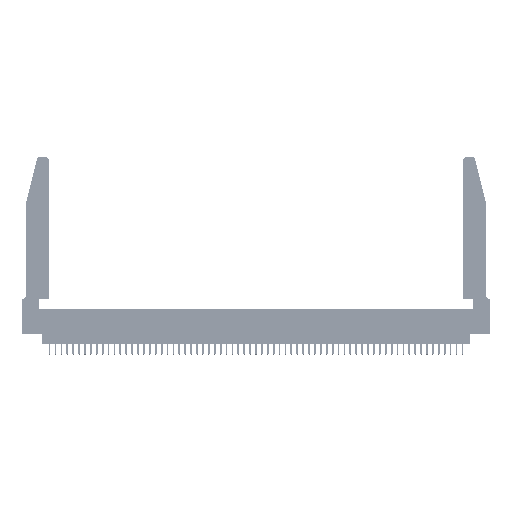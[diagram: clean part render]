
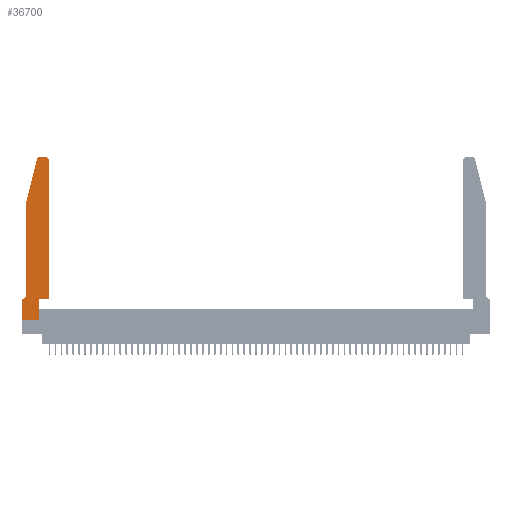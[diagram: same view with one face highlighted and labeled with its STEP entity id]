
A CAD part, top view. The second image highlights one B-rep face of the part: STEP entity #36700.
In plain terms, the highlighted planar face has unit normal (0, 0, 1).
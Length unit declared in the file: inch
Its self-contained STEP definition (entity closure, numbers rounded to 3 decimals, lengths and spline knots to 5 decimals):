
#953 = CARTESIAN_POINT ( 'NONE',  ( 0.2865, 0.35, 0.37 ) ) ;
#1869 = DIRECTION ( 'NONE',  ( 0., 0., 1. ) ) ;
#2263 = ORIENTED_EDGE ( 'NONE', *, *, #51978, .T. ) ;
#2476 = CARTESIAN_POINT ( 'NONE',  ( 0.0755, 2., 0.37 ) ) ;
#2962 = EDGE_CURVE ( 'NONE', #43943, #24867, #7674, .T. ) ;
#3345 = LINE ( 'NONE', #11328, #40398 ) ;
#3544 = EDGE_CURVE ( 'NONE', #31017, #8920, #23420, .T. ) ;
#3588 = VERTEX_POINT ( 'NONE', #51928 ) ;
#3883 = LINE ( 'NONE', #42548, #52692 ) ;
#4078 = ORIENTED_EDGE ( 'NONE', *, *, #52230, .T. ) ;
#4476 = LINE ( 'NONE', #19630, #51867 ) ;
#6431 = EDGE_LOOP ( 'NONE', ( #4078, #2263, #52543, #18265, #25940, #31523, #36903, #30570, #8687, #23156, #23454, #7984 ) ) ;
#7514 = AXIS2_PLACEMENT_3D ( 'NONE', #26543, #22287, #53197 ) ;
#7674 = LINE ( 'NONE', #29128, #52996 ) ;
#7984 = ORIENTED_EDGE ( 'NONE', *, *, #49078, .T. ) ;
#8687 = ORIENTED_EDGE ( 'NONE', *, *, #38161, .T. ) ;
#8920 = VERTEX_POINT ( 'NONE', #56820 ) ;
#10149 = AXIS2_PLACEMENT_3D ( 'NONE', #55018, #1869, #24113 ) ;
#10168 = AXIS2_PLACEMENT_3D ( 'NONE', #50578, #32696, #54780 ) ;
#10379 = VECTOR ( 'NONE', #34046, 39.37008 ) ;
#10678 = DIRECTION ( 'NONE',  ( 1., 0., 0. ) ) ;
#11328 = CARTESIAN_POINT ( 'NONE',  ( 0.2865, 0.35, 0.37 ) ) ;
#12524 = EDGE_CURVE ( 'NONE', #33496, #15859, #43593, .T. ) ;
#12536 = EDGE_CURVE ( 'NONE', #15859, #3588, #37429, .T. ) ;
#14085 = CARTESIAN_POINT ( 'NONE',  ( 0., 0., 0.37 ) ) ;
#14620 = AXIS2_PLACEMENT_3D ( 'NONE', #32933, #36957, #10678 ) ;
#14712 = VERTEX_POINT ( 'NONE', #953 ) ;
#15438 = EDGE_CURVE ( 'NONE', #22731, #39169, #36406, .T. ) ;
#15859 = VERTEX_POINT ( 'NONE', #52670 ) ;
#15919 = CARTESIAN_POINT ( 'NONE',  ( 0.2865, 0., 0.37 ) ) ;
#17232 = FACE_OUTER_BOUND ( 'NONE', #6431, .T. ) ;
#17410 = EDGE_CURVE ( 'NONE', #14712, #31017, #3883, .T. ) ;
#17604 = CARTESIAN_POINT ( 'NONE',  ( 0.0755, 0.42, 0.37 ) ) ;
#18265 = ORIENTED_EDGE ( 'NONE', *, *, #39097, .T. ) ;
#18310 = CIRCLE ( 'NONE', #10168, 0.03 ) ;
#19630 = CARTESIAN_POINT ( 'NONE',  ( 0., 0., 0.37 ) ) ;
#22086 = VERTEX_POINT ( 'NONE', #50207 ) ;
#22287 = DIRECTION ( 'NONE',  ( 0., 0., -1. ) ) ;
#22731 = VERTEX_POINT ( 'NONE', #14085 ) ;
#23156 = ORIENTED_EDGE ( 'NONE', *, *, #17410, .T. ) ;
#23420 = LINE ( 'NONE', #29648, #10379 ) ;
#23454 = ORIENTED_EDGE ( 'NONE', *, *, #3544, .T. ) ;
#24026 = DIRECTION ( 'NONE',  ( 0., -1., 0. ) ) ;
#24113 = DIRECTION ( 'NONE',  ( 1., 0., 0. ) ) ;
#24546 = DIRECTION ( 'NONE',  ( 0., -1., 0. ) ) ;
#24754 = VECTOR ( 'NONE', #36559, 39.37008 ) ;
#24758 = DIRECTION ( 'NONE',  ( 0., 1., 0. ) ) ;
#24867 = VERTEX_POINT ( 'NONE', #30318 ) ;
#25940 = ORIENTED_EDGE ( 'NONE', *, *, #12524, .T. ) ;
#26391 = CARTESIAN_POINT ( 'NONE',  ( 0.2605, 2.75, 0.37 ) ) ;
#26543 = CARTESIAN_POINT ( 'NONE',  ( 0.0055, 0.42, 0.37 ) ) ;
#26551 = VECTOR ( 'NONE', #24546, 39.37008 ) ;
#27164 = VECTOR ( 'NONE', #39371, 39.37008 ) ;
#28107 = CARTESIAN_POINT ( 'NONE',  ( 0.4505, 0.35, 0.37 ) ) ;
#28170 = PLANE ( 'NONE',  #10149 ) ;
#29128 = CARTESIAN_POINT ( 'NONE',  ( 0.0755, 2., 0.37 ) ) ;
#29648 = CARTESIAN_POINT ( 'NONE',  ( 0.4505, 0.35, 0.37 ) ) ;
#30318 = CARTESIAN_POINT ( 'NONE',  ( 0.0755, 2., 0.37 ) ) ;
#30570 = ORIENTED_EDGE ( 'NONE', *, *, #15438, .T. ) ;
#31017 = VERTEX_POINT ( 'NONE', #28107 ) ;
#31523 = ORIENTED_EDGE ( 'NONE', *, *, #12536, .T. ) ;
#32696 = DIRECTION ( 'NONE',  ( 0., 0., 1. ) ) ;
#32933 = CARTESIAN_POINT ( 'NONE',  ( 0.284, 2.72, 0.37 ) ) ;
#33095 = VERTEX_POINT ( 'NONE', #40467 ) ;
#33496 = VERTEX_POINT ( 'NONE', #17604 ) ;
#34046 = DIRECTION ( 'NONE',  ( 0., 1., 0. ) ) ;
#35190 = DIRECTION ( 'NONE',  ( -1., 0., 0. ) ) ;
#36406 = LINE ( 'NONE', #45381, #24754 ) ;
#36559 = DIRECTION ( 'NONE',  ( 1., 0., 0. ) ) ;
#36700 = ADVANCED_FACE ( 'NONE', ( #17232 ), #28170, .T. ) ;
#36903 = ORIENTED_EDGE ( 'NONE', *, *, #42087, .T. ) ;
#36957 = DIRECTION ( 'NONE',  ( 0., 0., 1. ) ) ;
#37429 = LINE ( 'NONE', #38436, #27164 ) ;
#38161 = EDGE_CURVE ( 'NONE', #39169, #14712, #3345, .T. ) ;
#38205 = LINE ( 'NONE', #2476, #26551 ) ;
#38436 = CARTESIAN_POINT ( 'NONE',  ( 0.0755, 0.35, 0.37 ) ) ;
#39097 = EDGE_CURVE ( 'NONE', #24867, #33496, #38205, .T. ) ;
#39169 = VERTEX_POINT ( 'NONE', #15919 ) ;
#39371 = DIRECTION ( 'NONE',  ( -1., 0., 0. ) ) ;
#40398 = VECTOR ( 'NONE', #24758, 39.37008 ) ;
#40467 = CARTESIAN_POINT ( 'NONE',  ( 0.284, 2.75, 0.37 ) ) ;
#42056 = VECTOR ( 'NONE', #35190, 39.37008 ) ;
#42087 = EDGE_CURVE ( 'NONE', #3588, #22731, #4476, .T. ) ;
#42548 = CARTESIAN_POINT ( 'NONE',  ( 0.4505, 0.35, 0.37 ) ) ;
#43593 = CIRCLE ( 'NONE', #7514, 0.07 ) ;
#43943 = VERTEX_POINT ( 'NONE', #46257 ) ;
#45381 = CARTESIAN_POINT ( 'NONE',  ( 0., 0., 0.37 ) ) ;
#46257 = CARTESIAN_POINT ( 'NONE',  ( 0.25487, 2.72718, 0.37 ) ) ;
#48938 = CIRCLE ( 'NONE', #14620, 0.03 ) ;
#49078 = EDGE_CURVE ( 'NONE', #8920, #22086, #18310, .T. ) ;
#50207 = CARTESIAN_POINT ( 'NONE',  ( 0.4205, 2.75, 0.37 ) ) ;
#50578 = CARTESIAN_POINT ( 'NONE',  ( 0.4205, 2.72, 0.37 ) ) ;
#51775 = DIRECTION ( 'NONE',  ( 1., 0., 0. ) ) ;
#51867 = VECTOR ( 'NONE', #24026, 39.37008 ) ;
#51928 = CARTESIAN_POINT ( 'NONE',  ( 0., 0.35, 0.37 ) ) ;
#51978 = EDGE_CURVE ( 'NONE', #33095, #43943, #48938, .T. ) ;
#52230 = EDGE_CURVE ( 'NONE', #22086, #33095, #53738, .T. ) ;
#52543 = ORIENTED_EDGE ( 'NONE', *, *, #2962, .T. ) ;
#52670 = CARTESIAN_POINT ( 'NONE',  ( 0.0055, 0.35, 0.37 ) ) ;
#52692 = VECTOR ( 'NONE', #51775, 39.37008 ) ;
#52996 = VECTOR ( 'NONE', #55782, 39.37008 ) ;
#53197 = DIRECTION ( 'NONE',  ( -1., 0., 0. ) ) ;
#53738 = LINE ( 'NONE', #26391, #42056 ) ;
#54780 = DIRECTION ( 'NONE',  ( 1., 0., 0. ) ) ;
#55018 = CARTESIAN_POINT ( 'NONE',  ( 0., 0.35, 0.37 ) ) ;
#55782 = DIRECTION ( 'NONE',  ( -0.239, -0.971, 0. ) ) ;
#56820 = CARTESIAN_POINT ( 'NONE',  ( 0.4505, 2.72, 0.37 ) ) ;
